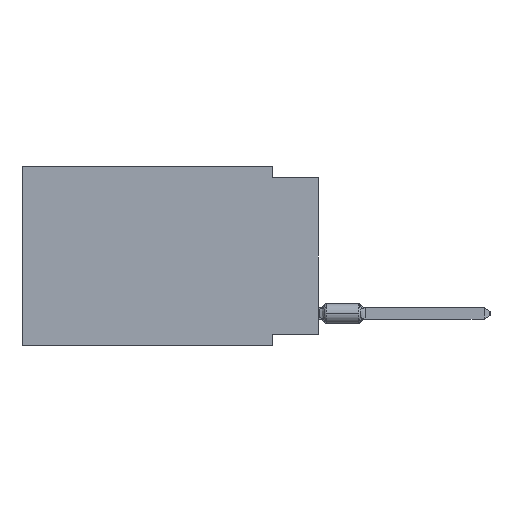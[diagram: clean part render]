
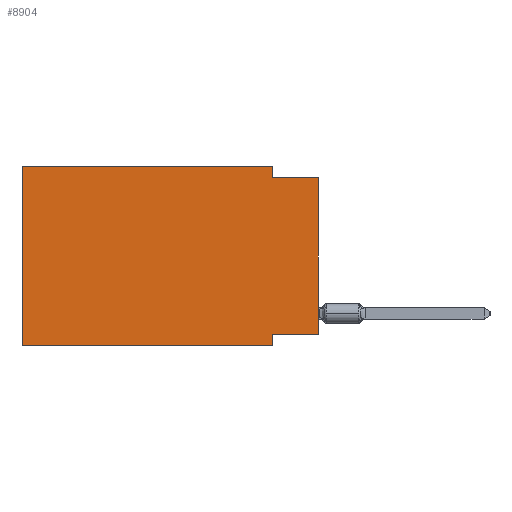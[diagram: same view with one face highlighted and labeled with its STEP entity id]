
A CAD part, left-side view. The second image highlights one B-rep face of the part: STEP entity #8904.
In plain terms, the highlighted planar face has unit normal (-1, 0, 0).
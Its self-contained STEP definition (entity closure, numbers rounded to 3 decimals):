
#2604 = ORIENTED_EDGE ( 'NONE', *, *, #66966, .F. ) ;
#2873 = DIRECTION ( 'NONE',  ( 0., -1., 0. ) ) ;
#3566 = DIRECTION ( 'NONE',  ( 0., 0., 1. ) ) ;
#4236 = PLANE ( 'NONE',  #19168 ) ;
#5489 = DIRECTION ( 'NONE',  ( 0., 0., -1. ) ) ;
#5549 = CARTESIAN_POINT ( 'NONE',  ( 0., 0., -9.271 ) ) ;
#7406 = EDGE_CURVE ( 'NONE', #59660, #57702, #55796, .T. ) ;
#7793 = CARTESIAN_POINT ( 'NONE',  ( 0., 0., -0.635 ) ) ;
#8517 = LINE ( 'NONE', #37835, #23575 ) ;
#8543 = LINE ( 'NONE', #7793, #25154 ) ;
#8904 = ADVANCED_FACE ( 'NONE', ( #39579 ), #4236, .F. ) ;
#10389 = VERTEX_POINT ( 'NONE', #43299 ) ;
#10478 = VERTEX_POINT ( 'NONE', #45880 ) ;
#11898 = VECTOR ( 'NONE', #21414, 1000. ) ;
#12133 = ORIENTED_EDGE ( 'NONE', *, *, #63112, .T. ) ;
#15560 = EDGE_LOOP ( 'NONE', ( #67222, #36034, #56041, #56094, #70792, #12133, #2604, #43569 ) ) ;
#15774 = DIRECTION ( 'NONE',  ( 0., 0., -1. ) ) ;
#19168 = AXIS2_PLACEMENT_3D ( 'NONE', #62536, #33935, #56538 ) ;
#21146 = DIRECTION ( 'NONE',  ( 0., 1., 0. ) ) ;
#21414 = DIRECTION ( 'NONE',  ( 0., 0., 1. ) ) ;
#21418 = LINE ( 'NONE', #44378, #55836 ) ;
#23575 = VECTOR ( 'NONE', #2873, 1000. ) ;
#24079 = CARTESIAN_POINT ( 'NONE',  ( 0., 16.383, 0. ) ) ;
#25154 = VECTOR ( 'NONE', #26209, 1000. ) ;
#25389 = CARTESIAN_POINT ( 'NONE',  ( 0., 16.383, 0. ) ) ;
#26209 = DIRECTION ( 'NONE',  ( 0., -1., 0. ) ) ;
#26721 = VERTEX_POINT ( 'NONE', #69559 ) ;
#26792 = CARTESIAN_POINT ( 'NONE',  ( 0., 16.383, 0. ) ) ;
#29314 = EDGE_CURVE ( 'NONE', #64400, #42462, #21418, .T. ) ;
#29965 = VECTOR ( 'NONE', #21146, 1000. ) ;
#31032 = LINE ( 'NONE', #25389, #70357 ) ;
#31223 = VECTOR ( 'NONE', #5489, 1000. ) ;
#32959 = LINE ( 'NONE', #34080, #31223 ) ;
#33935 = DIRECTION ( 'NONE',  ( 1., 0., 0. ) ) ;
#34080 = CARTESIAN_POINT ( 'NONE',  ( 0., 2.54, -9.906 ) ) ;
#34746 = EDGE_CURVE ( 'NONE', #42462, #10389, #8543, .T. ) ;
#34964 = VERTEX_POINT ( 'NONE', #24079 ) ;
#36034 = ORIENTED_EDGE ( 'NONE', *, *, #34746, .F. ) ;
#37488 = EDGE_CURVE ( 'NONE', #34964, #64400, #50870, .T. ) ;
#37722 = CARTESIAN_POINT ( 'NONE',  ( 0., 0., -9.271 ) ) ;
#37835 = CARTESIAN_POINT ( 'NONE',  ( 0., 16.383, -9.906 ) ) ;
#38834 = DIRECTION ( 'NONE',  ( 0., -1., 0. ) ) ;
#39579 = FACE_OUTER_BOUND ( 'NONE', #15560, .T. ) ;
#39843 = CARTESIAN_POINT ( 'NONE',  ( 0., 0., 0. ) ) ;
#42462 = VERTEX_POINT ( 'NONE', #50868 ) ;
#43299 = CARTESIAN_POINT ( 'NONE',  ( 0., 0., -0.635 ) ) ;
#43569 = ORIENTED_EDGE ( 'NONE', *, *, #7406, .F. ) ;
#44378 = CARTESIAN_POINT ( 'NONE',  ( 0., 2.54, 0. ) ) ;
#44917 = CARTESIAN_POINT ( 'NONE',  ( 0., 2.54, -9.271 ) ) ;
#45880 = CARTESIAN_POINT ( 'NONE',  ( 0., 2.54, -9.906 ) ) ;
#50026 = LINE ( 'NONE', #39843, #11898 ) ;
#50733 = EDGE_CURVE ( 'NONE', #26721, #34964, #31032, .T. ) ;
#50868 = CARTESIAN_POINT ( 'NONE',  ( 0., 2.54, -0.635 ) ) ;
#50870 = LINE ( 'NONE', #26792, #57875 ) ;
#51006 = CARTESIAN_POINT ( 'NONE',  ( 0., 2.54, 0. ) ) ;
#55743 = EDGE_CURVE ( 'NONE', #59660, #10389, #50026, .T. ) ;
#55796 = LINE ( 'NONE', #37722, #29965 ) ;
#55836 = VECTOR ( 'NONE', #15774, 1000. ) ;
#56041 = ORIENTED_EDGE ( 'NONE', *, *, #29314, .F. ) ;
#56094 = ORIENTED_EDGE ( 'NONE', *, *, #37488, .F. ) ;
#56538 = DIRECTION ( 'NONE',  ( 0., 0., -1. ) ) ;
#57702 = VERTEX_POINT ( 'NONE', #44917 ) ;
#57875 = VECTOR ( 'NONE', #38834, 1000. ) ;
#59660 = VERTEX_POINT ( 'NONE', #5549 ) ;
#62536 = CARTESIAN_POINT ( 'NONE',  ( 0., 16.383, 0. ) ) ;
#63112 = EDGE_CURVE ( 'NONE', #26721, #10478, #8517, .T. ) ;
#64400 = VERTEX_POINT ( 'NONE', #51006 ) ;
#66966 = EDGE_CURVE ( 'NONE', #57702, #10478, #32959, .T. ) ;
#67222 = ORIENTED_EDGE ( 'NONE', *, *, #55743, .T. ) ;
#69559 = CARTESIAN_POINT ( 'NONE',  ( 0., 16.383, -9.906 ) ) ;
#70357 = VECTOR ( 'NONE', #3566, 1000. ) ;
#70792 = ORIENTED_EDGE ( 'NONE', *, *, #50733, .F. ) ;
